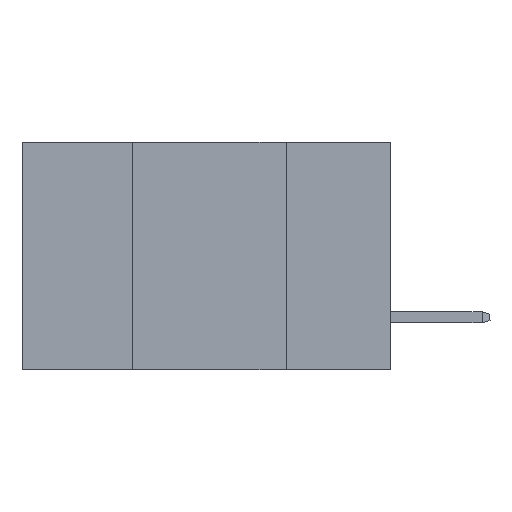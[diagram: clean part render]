
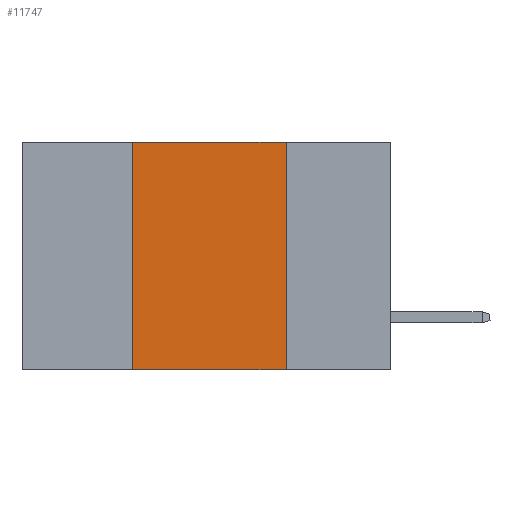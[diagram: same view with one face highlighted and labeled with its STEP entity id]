
A CAD part, left-side view. The second image highlights one B-rep face of the part: STEP entity #11747.
In plain terms, the highlighted planar face has unit normal (-1, 0, 0).
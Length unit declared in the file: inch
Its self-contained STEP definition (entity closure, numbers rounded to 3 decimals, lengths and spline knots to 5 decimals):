
#116 = EDGE_CURVE ( 'NONE', #8579, #12469, #2111, .T. ) ;
#1057 = DIRECTION ( 'NONE',  ( 0., 0., -1. ) ) ;
#1318 = ORIENTED_EDGE ( 'NONE', *, *, #3450, .F. ) ;
#1510 = CARTESIAN_POINT ( 'NONE',  ( 0., 0.17, 0. ) ) ;
#1718 = ORIENTED_EDGE ( 'NONE', *, *, #7150, .F. ) ;
#2062 = ORIENTED_EDGE ( 'NONE', *, *, #116, .F. ) ;
#2111 = LINE ( 'NONE', #9419, #13653 ) ;
#2223 = DIRECTION ( 'NONE',  ( 1., 0., 0. ) ) ;
#2472 = CARTESIAN_POINT ( 'NONE',  ( 0., 0.17, -0.37 ) ) ;
#3105 = VECTOR ( 'NONE', #3419, 39.37008 ) ;
#3168 = CARTESIAN_POINT ( 'NONE',  ( 0., 0.6, 0. ) ) ;
#3419 = DIRECTION ( 'NONE',  ( 0., 0., -1. ) ) ;
#3428 = CARTESIAN_POINT ( 'NONE',  ( 0., 0.6, -0.37 ) ) ;
#3450 = EDGE_CURVE ( 'NONE', #13288, #8579, #4769, .T. ) ;
#4288 = DIRECTION ( 'NONE',  ( 0., 0., 1. ) ) ;
#4642 = DIRECTION ( 'NONE',  ( 0., -1., 0. ) ) ;
#4769 = LINE ( 'NONE', #11001, #11005 ) ;
#4933 = LINE ( 'NONE', #3428, #13865 ) ;
#4935 = EDGE_LOOP ( 'NONE', ( #1718, #2062, #1318, #6160 ) ) ;
#4982 = VERTEX_POINT ( 'NONE', #2472 ) ;
#5679 = CARTESIAN_POINT ( 'NONE',  ( 0., 0.42, -0.37 ) ) ;
#5799 = EDGE_CURVE ( 'NONE', #13288, #4982, #4933, .T. ) ;
#6160 = ORIENTED_EDGE ( 'NONE', *, *, #5799, .T. ) ;
#6601 = PLANE ( 'NONE',  #14042 ) ;
#6926 = CARTESIAN_POINT ( 'NONE',  ( 0., 0.17, 0. ) ) ;
#7150 = EDGE_CURVE ( 'NONE', #12469, #4982, #8182, .T. ) ;
#8168 = DIRECTION ( 'NONE',  ( 0., -1., 0. ) ) ;
#8182 = LINE ( 'NONE', #6926, #3105 ) ;
#8579 = VERTEX_POINT ( 'NONE', #13217 ) ;
#9219 = FACE_OUTER_BOUND ( 'NONE', #4935, .T. ) ;
#9419 = CARTESIAN_POINT ( 'NONE',  ( 0., 0.6, 0. ) ) ;
#11001 = CARTESIAN_POINT ( 'NONE',  ( 0., 0.42, 0. ) ) ;
#11005 = VECTOR ( 'NONE', #4288, 39.37008 ) ;
#11747 = ADVANCED_FACE ( 'NONE', ( #9219 ), #6601, .F. ) ;
#12469 = VERTEX_POINT ( 'NONE', #1510 ) ;
#13217 = CARTESIAN_POINT ( 'NONE',  ( 0., 0.42, 0. ) ) ;
#13288 = VERTEX_POINT ( 'NONE', #5679 ) ;
#13653 = VECTOR ( 'NONE', #8168, 39.37008 ) ;
#13865 = VECTOR ( 'NONE', #4642, 39.37008 ) ;
#14042 = AXIS2_PLACEMENT_3D ( 'NONE', #3168, #2223, #1057 ) ;
